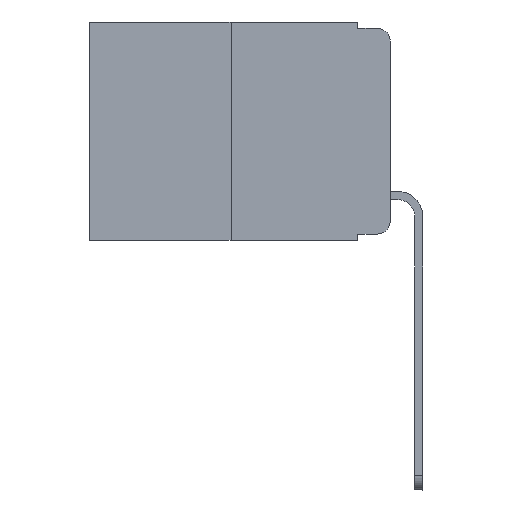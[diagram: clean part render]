
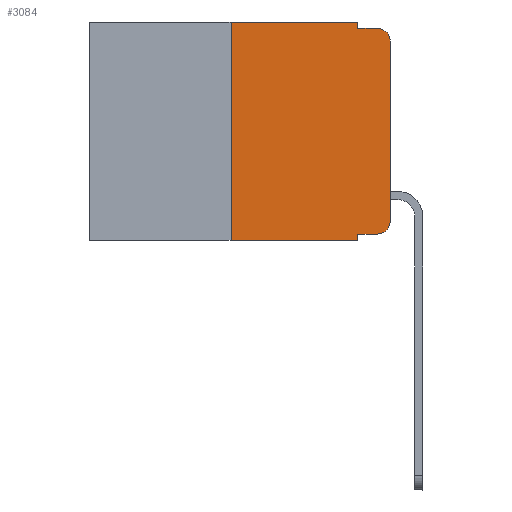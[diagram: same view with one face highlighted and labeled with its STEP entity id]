
A CAD part, left-side view. The second image highlights one B-rep face of the part: STEP entity #3084.
In plain terms, the highlighted planar face has unit normal (-1, 0, 0).
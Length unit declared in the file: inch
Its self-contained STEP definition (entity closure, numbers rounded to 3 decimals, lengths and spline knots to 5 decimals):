
#1429 = ORIENTED_EDGE ( 'NONE', *, *, #11860, .F. ) ;
#1590 = CARTESIAN_POINT ( 'NONE',  ( 0., 0., -0.03 ) ) ;
#1632 = EDGE_CURVE ( 'NONE', #4209, #15463, #2797, .T. ) ;
#1691 = VECTOR ( 'NONE', #10210, 39.37008 ) ;
#2797 = CIRCLE ( 'NONE', #15586, 0.02 ) ;
#2916 = CARTESIAN_POINT ( 'NONE',  ( 0., 0.051, -0.01 ) ) ;
#3049 = VECTOR ( 'NONE', #12794, 39.37008 ) ;
#3084 = ADVANCED_FACE ( 'NONE', ( #19165 ), #12100, .F. ) ;
#3529 = DIRECTION ( 'NONE',  ( 0., -1., 0. ) ) ;
#3540 = DIRECTION ( 'NONE',  ( 0., 0., -1. ) ) ;
#4209 = VERTEX_POINT ( 'NONE', #9435 ) ;
#4243 = CARTESIAN_POINT ( 'NONE',  ( 0., 0.473, 0. ) ) ;
#4332 = EDGE_CURVE ( 'NONE', #19843, #11881, #20277, .T. ) ;
#4660 = LINE ( 'NONE', #18088, #7310 ) ;
#4828 = CARTESIAN_POINT ( 'NONE',  ( 0., 0.051, 0. ) ) ;
#4944 = LINE ( 'NONE', #4828, #10922 ) ;
#4965 = VERTEX_POINT ( 'NONE', #7581 ) ;
#5091 = CARTESIAN_POINT ( 'NONE',  ( 0., 0.473, -0.343 ) ) ;
#5318 = CARTESIAN_POINT ( 'NONE',  ( 0., 0.473, 0. ) ) ;
#5379 = DIRECTION ( 'NONE',  ( -1., 0., 0. ) ) ;
#5731 = DIRECTION ( 'NONE',  ( 1., 0., 0. ) ) ;
#5807 = VECTOR ( 'NONE', #3540, 39.37008 ) ;
#5825 = CARTESIAN_POINT ( 'NONE',  ( 0., 0.051, -0.01 ) ) ;
#5832 = CARTESIAN_POINT ( 'NONE',  ( 0., 0.25, 0. ) ) ;
#6033 = CARTESIAN_POINT ( 'NONE',  ( 0., 0.051, 0. ) ) ;
#6099 = ORIENTED_EDGE ( 'NONE', *, *, #1632, .T. ) ;
#6236 = VECTOR ( 'NONE', #12709, 39.37008 ) ;
#6398 = ORIENTED_EDGE ( 'NONE', *, *, #8108, .F. ) ;
#6644 = EDGE_LOOP ( 'NONE', ( #14165, #17503, #9820, #1429, #6398, #18778, #13750, #14313, #10890, #6099 ) ) ;
#6677 = VERTEX_POINT ( 'NONE', #1590 ) ;
#7092 = EDGE_CURVE ( 'NONE', #11671, #11881, #9964, .T. ) ;
#7247 = CARTESIAN_POINT ( 'NONE',  ( 0., 0.25, 0. ) ) ;
#7310 = VECTOR ( 'NONE', #11670, 39.37008 ) ;
#7433 = AXIS2_PLACEMENT_3D ( 'NONE', #5318, #5731, #8965 ) ;
#7581 = CARTESIAN_POINT ( 'NONE',  ( 0., 0.02, -0.01 ) ) ;
#8011 = LINE ( 'NONE', #2916, #6236 ) ;
#8108 = EDGE_CURVE ( 'NONE', #11891, #20890, #11099, .T. ) ;
#8272 = AXIS2_PLACEMENT_3D ( 'NONE', #11731, #5379, #12284 ) ;
#8502 = CARTESIAN_POINT ( 'NONE',  ( 0., 0.051, -0.333 ) ) ;
#8965 = DIRECTION ( 'NONE',  ( 0., 0., -1. ) ) ;
#8999 = CIRCLE ( 'NONE', #8272, 0.02 ) ;
#9288 = LINE ( 'NONE', #5832, #9382 ) ;
#9382 = VECTOR ( 'NONE', #19374, 39.37008 ) ;
#9435 = CARTESIAN_POINT ( 'NONE',  ( 0., 0.02, -0.333 ) ) ;
#9820 = ORIENTED_EDGE ( 'NONE', *, *, #21306, .F. ) ;
#9964 = LINE ( 'NONE', #18504, #5807 ) ;
#10210 = DIRECTION ( 'NONE',  ( 0., -1., 0. ) ) ;
#10242 = VERTEX_POINT ( 'NONE', #5825 ) ;
#10380 = LINE ( 'NONE', #8502, #14706 ) ;
#10733 = CARTESIAN_POINT ( 'NONE',  ( 0., 0.051, -0.333 ) ) ;
#10890 = ORIENTED_EDGE ( 'NONE', *, *, #18510, .T. ) ;
#10922 = VECTOR ( 'NONE', #11622, 39.37008 ) ;
#11099 = LINE ( 'NONE', #4243, #3049 ) ;
#11622 = DIRECTION ( 'NONE',  ( 0., 0., -1. ) ) ;
#11670 = DIRECTION ( 'NONE',  ( 0., 0., 1. ) ) ;
#11671 = VERTEX_POINT ( 'NONE', #10733 ) ;
#11731 = CARTESIAN_POINT ( 'NONE',  ( 0., 0.02, -0.03 ) ) ;
#11860 = EDGE_CURVE ( 'NONE', #20890, #10242, #4944, .T. ) ;
#11877 = EDGE_CURVE ( 'NONE', #6677, #4965, #8999, .T. ) ;
#11881 = VERTEX_POINT ( 'NONE', #20568 ) ;
#11891 = VERTEX_POINT ( 'NONE', #7247 ) ;
#12100 = PLANE ( 'NONE',  #7433 ) ;
#12284 = DIRECTION ( 'NONE',  ( 0., 0., -1. ) ) ;
#12709 = DIRECTION ( 'NONE',  ( 0., -1., 0. ) ) ;
#12794 = DIRECTION ( 'NONE',  ( 0., -1., 0. ) ) ;
#13406 = CARTESIAN_POINT ( 'NONE',  ( 0., 0., -0.313 ) ) ;
#13750 = ORIENTED_EDGE ( 'NONE', *, *, #4332, .T. ) ;
#14056 = CARTESIAN_POINT ( 'NONE',  ( 0., 0.25, -0.343 ) ) ;
#14165 = ORIENTED_EDGE ( 'NONE', *, *, #19955, .T. ) ;
#14170 = CARTESIAN_POINT ( 'NONE',  ( 0., 0.02, -0.313 ) ) ;
#14313 = ORIENTED_EDGE ( 'NONE', *, *, #7092, .F. ) ;
#14706 = VECTOR ( 'NONE', #3529, 39.37008 ) ;
#15463 = VERTEX_POINT ( 'NONE', #13406 ) ;
#15586 = AXIS2_PLACEMENT_3D ( 'NONE', #14170, #20886, #16023 ) ;
#16023 = DIRECTION ( 'NONE',  ( 0., 0., -1. ) ) ;
#17503 = ORIENTED_EDGE ( 'NONE', *, *, #11877, .T. ) ;
#18088 = CARTESIAN_POINT ( 'NONE',  ( 0., 0., 0. ) ) ;
#18342 = EDGE_CURVE ( 'NONE', #19843, #11891, #9288, .T. ) ;
#18504 = CARTESIAN_POINT ( 'NONE',  ( 0., 0.051, 0. ) ) ;
#18510 = EDGE_CURVE ( 'NONE', #11671, #4209, #10380, .T. ) ;
#18778 = ORIENTED_EDGE ( 'NONE', *, *, #18342, .F. ) ;
#19165 = FACE_OUTER_BOUND ( 'NONE', #6644, .T. ) ;
#19374 = DIRECTION ( 'NONE',  ( 0., 0., 1. ) ) ;
#19843 = VERTEX_POINT ( 'NONE', #14056 ) ;
#19955 = EDGE_CURVE ( 'NONE', #15463, #6677, #4660, .T. ) ;
#20277 = LINE ( 'NONE', #5091, #1691 ) ;
#20568 = CARTESIAN_POINT ( 'NONE',  ( 0., 0.051, -0.343 ) ) ;
#20886 = DIRECTION ( 'NONE',  ( -1., 0., 0. ) ) ;
#20890 = VERTEX_POINT ( 'NONE', #6033 ) ;
#21306 = EDGE_CURVE ( 'NONE', #10242, #4965, #8011, .T. ) ;
